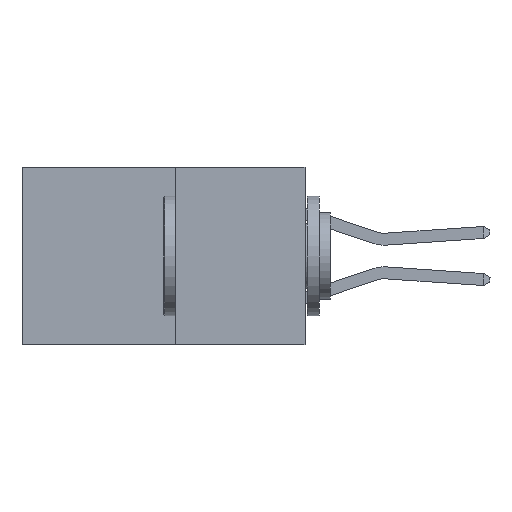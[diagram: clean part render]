
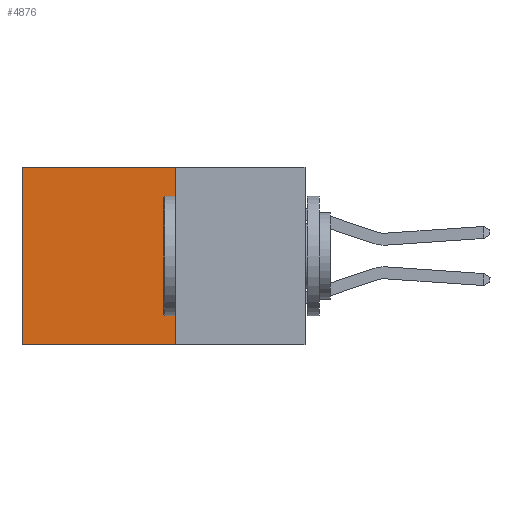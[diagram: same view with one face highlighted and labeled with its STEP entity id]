
A CAD part, left-side view. The second image highlights one B-rep face of the part: STEP entity #4876.
In plain terms, the highlighted planar face has unit normal (-1, 0, 0).
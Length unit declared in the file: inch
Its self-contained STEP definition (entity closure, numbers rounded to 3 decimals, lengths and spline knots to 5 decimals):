
#684 = VERTEX_POINT ( 'NONE', #1134 ) ;
#691 = CARTESIAN_POINT ( 'NONE',  ( 0.277, 0.27, 0. ) ) ;
#1134 = CARTESIAN_POINT ( 'NONE',  ( 0.277, 0.27, -0.37 ) ) ;
#1165 = CARTESIAN_POINT ( 'NONE',  ( 0.277, 0.27, -0.37 ) ) ;
#1479 = VERTEX_POINT ( 'NONE', #9125 ) ;
#1545 = VECTOR ( 'NONE', #5500, 39.37008 ) ;
#1635 = LINE ( 'NONE', #691, #5904 ) ;
#2491 = VECTOR ( 'NONE', #3457, 39.37008 ) ;
#2692 = CARTESIAN_POINT ( 'NONE',  ( 0.277, 0.59, -0.37 ) ) ;
#3214 = DIRECTION ( 'NONE',  ( 1., 0., 0. ) ) ;
#3457 = DIRECTION ( 'NONE',  ( 0., 1., 0. ) ) ;
#3522 = CARTESIAN_POINT ( 'NONE',  ( 0.277, 0.27, -0.37 ) ) ;
#3877 = LINE ( 'NONE', #1165, #1545 ) ;
#3918 = VECTOR ( 'NONE', #9296, 39.37008 ) ;
#4477 = EDGE_CURVE ( 'NONE', #684, #6030, #4744, .T. ) ;
#4744 = LINE ( 'NONE', #3522, #2491 ) ;
#4876 = ADVANCED_FACE ( 'NONE', ( #6690 ), #10377, .F. ) ;
#4964 = EDGE_CURVE ( 'NONE', #1479, #10472, #1635, .T. ) ;
#5071 = DIRECTION ( 'NONE',  ( 0., 1., 0. ) ) ;
#5355 = CARTESIAN_POINT ( 'NONE',  ( 0.277, 0.59, -0.37 ) ) ;
#5500 = DIRECTION ( 'NONE',  ( 0., 0., -1. ) ) ;
#5904 = VECTOR ( 'NONE', #5071, 39.37008 ) ;
#6030 = VERTEX_POINT ( 'NONE', #2692 ) ;
#6161 = ORIENTED_EDGE ( 'NONE', *, *, #4964, .T. ) ;
#6415 = EDGE_LOOP ( 'NONE', ( #9327, #7752, #7994, #6161 ) ) ;
#6690 = FACE_OUTER_BOUND ( 'NONE', #6415, .T. ) ;
#6852 = AXIS2_PLACEMENT_3D ( 'NONE', #8105, #3214, #8876 ) ;
#7204 = EDGE_CURVE ( 'NONE', #10472, #6030, #8223, .T. ) ;
#7752 = ORIENTED_EDGE ( 'NONE', *, *, #4477, .F. ) ;
#7814 = CARTESIAN_POINT ( 'NONE',  ( 0.277, 0.59, 0. ) ) ;
#7994 = ORIENTED_EDGE ( 'NONE', *, *, #10554, .F. ) ;
#8105 = CARTESIAN_POINT ( 'NONE',  ( 0.277, 0.27, -0.37 ) ) ;
#8223 = LINE ( 'NONE', #5355, #3918 ) ;
#8876 = DIRECTION ( 'NONE',  ( 0., 0., -1. ) ) ;
#9125 = CARTESIAN_POINT ( 'NONE',  ( 0.277, 0.27, 0. ) ) ;
#9296 = DIRECTION ( 'NONE',  ( 0., 0., -1. ) ) ;
#9327 = ORIENTED_EDGE ( 'NONE', *, *, #7204, .T. ) ;
#10377 = PLANE ( 'NONE',  #6852 ) ;
#10472 = VERTEX_POINT ( 'NONE', #7814 ) ;
#10554 = EDGE_CURVE ( 'NONE', #1479, #684, #3877, .T. ) ;
